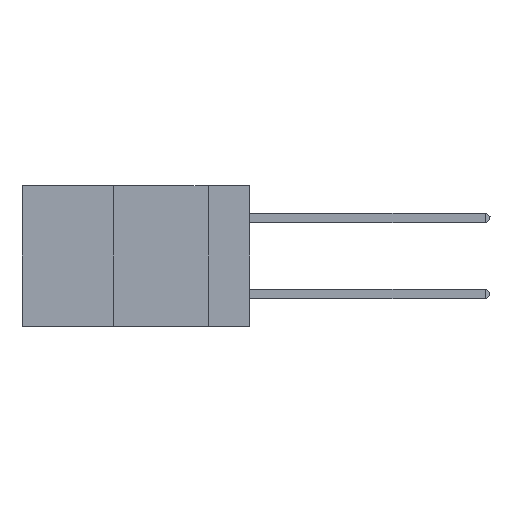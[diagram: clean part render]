
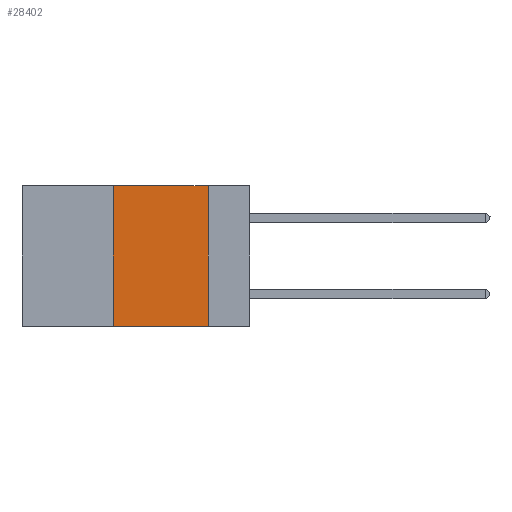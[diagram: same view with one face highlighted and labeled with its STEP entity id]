
A CAD part, left-side view. The second image highlights one B-rep face of the part: STEP entity #28402.
In plain terms, the highlighted planar face has unit normal (-1, 0, 0).
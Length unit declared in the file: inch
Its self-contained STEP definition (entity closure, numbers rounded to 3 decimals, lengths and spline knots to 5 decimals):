
#192 = CARTESIAN_POINT ( 'NONE',  ( 0., 0.6, -0.37 ) ) ;
#1728 = EDGE_LOOP ( 'NONE', ( #27500, #25365, #27541, #37327 ) ) ;
#1806 = CARTESIAN_POINT ( 'NONE',  ( 0., 0.11, -0.37 ) ) ;
#3187 = VERTEX_POINT ( 'NONE', #1806 ) ;
#4854 = AXIS2_PLACEMENT_3D ( 'NONE', #15978, #7068, #31811 ) ;
#4961 = EDGE_CURVE ( 'NONE', #32169, #12919, #18189, .T. ) ;
#6042 = CARTESIAN_POINT ( 'NONE',  ( 0., 0.36, -0.37 ) ) ;
#7068 = DIRECTION ( 'NONE',  ( 1., 0., 0. ) ) ;
#8090 = VERTEX_POINT ( 'NONE', #6042 ) ;
#8743 = LINE ( 'NONE', #35713, #22989 ) ;
#10519 = CARTESIAN_POINT ( 'NONE',  ( 0., 0.6, 0. ) ) ;
#10766 = CARTESIAN_POINT ( 'NONE',  ( 0., 0.36, 0. ) ) ;
#11299 = CARTESIAN_POINT ( 'NONE',  ( 0., 0.36, 0. ) ) ;
#12919 = VERTEX_POINT ( 'NONE', #33424 ) ;
#15978 = CARTESIAN_POINT ( 'NONE',  ( 0., 0.6, 0. ) ) ;
#17681 = EDGE_CURVE ( 'NONE', #12919, #3187, #8743, .T. ) ;
#18189 = LINE ( 'NONE', #10519, #23927 ) ;
#18634 = DIRECTION ( 'NONE',  ( 0., -1., 0. ) ) ;
#20902 = DIRECTION ( 'NONE',  ( 0., 0., -1. ) ) ;
#22989 = VECTOR ( 'NONE', #20902, 39.37008 ) ;
#23015 = LINE ( 'NONE', #192, #30203 ) ;
#23927 = VECTOR ( 'NONE', #33604, 39.37008 ) ;
#24707 = PLANE ( 'NONE',  #4854 ) ;
#25365 = ORIENTED_EDGE ( 'NONE', *, *, #4961, .F. ) ;
#26389 = EDGE_CURVE ( 'NONE', #8090, #32169, #32293, .T. ) ;
#27500 = ORIENTED_EDGE ( 'NONE', *, *, #17681, .F. ) ;
#27541 = ORIENTED_EDGE ( 'NONE', *, *, #26389, .F. ) ;
#28402 = ADVANCED_FACE ( 'NONE', ( #37089 ), #24707, .F. ) ;
#29980 = VECTOR ( 'NONE', #32702, 39.37008 ) ;
#30203 = VECTOR ( 'NONE', #18634, 39.37008 ) ;
#30810 = EDGE_CURVE ( 'NONE', #8090, #3187, #23015, .T. ) ;
#31811 = DIRECTION ( 'NONE',  ( 0., 0., -1. ) ) ;
#32169 = VERTEX_POINT ( 'NONE', #11299 ) ;
#32293 = LINE ( 'NONE', #10766, #29980 ) ;
#32702 = DIRECTION ( 'NONE',  ( 0., 0., 1. ) ) ;
#33424 = CARTESIAN_POINT ( 'NONE',  ( 0., 0.11, 0. ) ) ;
#33604 = DIRECTION ( 'NONE',  ( 0., -1., 0. ) ) ;
#35713 = CARTESIAN_POINT ( 'NONE',  ( 0., 0.11, 0. ) ) ;
#37089 = FACE_OUTER_BOUND ( 'NONE', #1728, .T. ) ;
#37327 = ORIENTED_EDGE ( 'NONE', *, *, #30810, .T. ) ;
